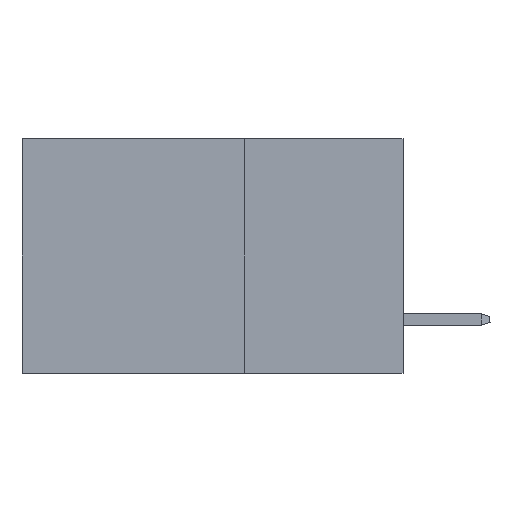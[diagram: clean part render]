
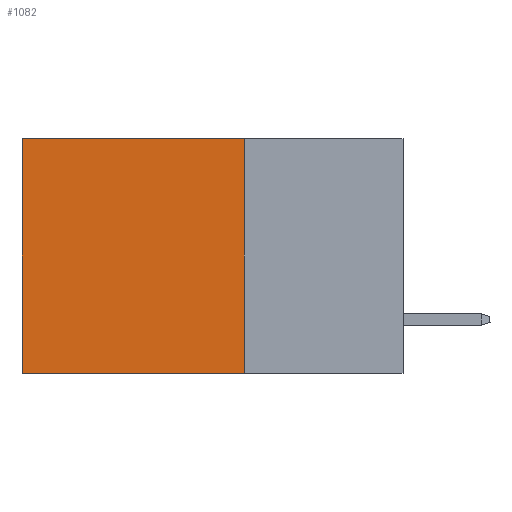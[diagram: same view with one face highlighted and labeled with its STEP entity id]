
A CAD part, left-side view. The second image highlights one B-rep face of the part: STEP entity #1082.
In plain terms, the highlighted planar face has unit normal (-1, 0, 0).
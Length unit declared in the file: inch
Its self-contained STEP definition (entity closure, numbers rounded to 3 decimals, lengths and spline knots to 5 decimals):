
#1082 = ADVANCED_FACE ( 'NONE', ( #13356 ), #10580, .F. ) ;
#2274 = VERTEX_POINT ( 'NONE', #34996 ) ;
#2595 = CARTESIAN_POINT ( 'NONE',  ( 0.2875, 0.6, 0. ) ) ;
#4135 = LINE ( 'NONE', #17147, #18286 ) ;
#5015 = VECTOR ( 'NONE', #6000, 39.37008 ) ;
#6000 = DIRECTION ( 'NONE',  ( 0., 0., -1. ) ) ;
#6020 = VECTOR ( 'NONE', #40768, 39.37008 ) ;
#6491 = DIRECTION ( 'NONE',  ( 0., 1., 0. ) ) ;
#6869 = ORIENTED_EDGE ( 'NONE', *, *, #27104, .F. ) ;
#8721 = ORIENTED_EDGE ( 'NONE', *, *, #34876, .T. ) ;
#8782 = CARTESIAN_POINT ( 'NONE',  ( 0.2875, 0.25, 0. ) ) ;
#8844 = VERTEX_POINT ( 'NONE', #10142 ) ;
#10007 = VERTEX_POINT ( 'NONE', #12923 ) ;
#10142 = CARTESIAN_POINT ( 'NONE',  ( 0.2875, 0.6, 0. ) ) ;
#10580 = PLANE ( 'NONE',  #41328 ) ;
#10791 = DIRECTION ( 'NONE',  ( 1., 0., 0. ) ) ;
#12923 = CARTESIAN_POINT ( 'NONE',  ( 0.2875, 0.25, -0.37 ) ) ;
#12977 = ORIENTED_EDGE ( 'NONE', *, *, #17053, .F. ) ;
#13356 = FACE_OUTER_BOUND ( 'NONE', #27947, .T. ) ;
#14573 = LINE ( 'NONE', #8782, #19310 ) ;
#16975 = CARTESIAN_POINT ( 'NONE',  ( 0.2875, 0.25, 0. ) ) ;
#17053 = EDGE_CURVE ( 'NONE', #18242, #10007, #14573, .T. ) ;
#17147 = CARTESIAN_POINT ( 'NONE',  ( 0.2875, 0.25, 0. ) ) ;
#17257 = EDGE_CURVE ( 'NONE', #8844, #2274, #29025, .T. ) ;
#17970 = DIRECTION ( 'NONE',  ( 0., 0., -1. ) ) ;
#18242 = VERTEX_POINT ( 'NONE', #40460 ) ;
#18286 = VECTOR ( 'NONE', #6491, 39.37008 ) ;
#19310 = VECTOR ( 'NONE', #17970, 39.37008 ) ;
#26365 = DIRECTION ( 'NONE',  ( 0., 0., -1. ) ) ;
#27104 = EDGE_CURVE ( 'NONE', #10007, #2274, #40555, .T. ) ;
#27947 = EDGE_LOOP ( 'NONE', ( #35105, #6869, #12977, #8721 ) ) ;
#29025 = LINE ( 'NONE', #2595, #5015 ) ;
#31351 = CARTESIAN_POINT ( 'NONE',  ( 0.2875, 0.25, -0.37 ) ) ;
#34876 = EDGE_CURVE ( 'NONE', #18242, #8844, #4135, .T. ) ;
#34996 = CARTESIAN_POINT ( 'NONE',  ( 0.2875, 0.6, -0.37 ) ) ;
#35105 = ORIENTED_EDGE ( 'NONE', *, *, #17257, .T. ) ;
#40460 = CARTESIAN_POINT ( 'NONE',  ( 0.2875, 0.25, 0. ) ) ;
#40555 = LINE ( 'NONE', #31351, #6020 ) ;
#40768 = DIRECTION ( 'NONE',  ( 0., 1., 0. ) ) ;
#41328 = AXIS2_PLACEMENT_3D ( 'NONE', #16975, #10791, #26365 ) ;
